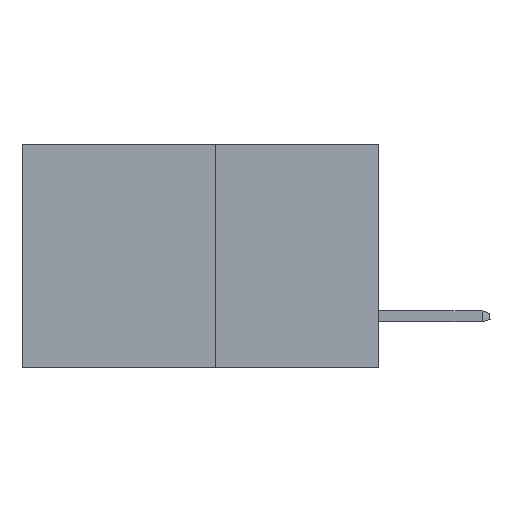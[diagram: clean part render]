
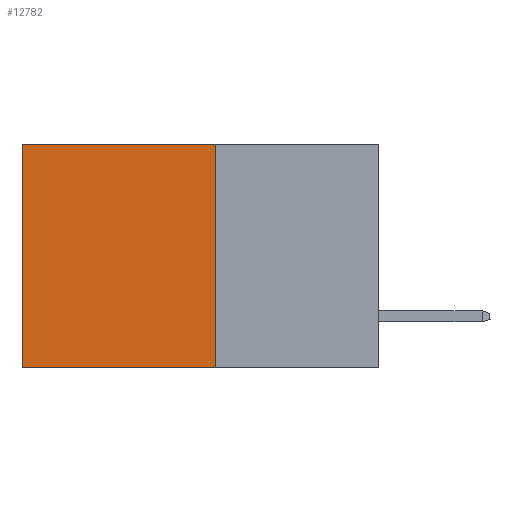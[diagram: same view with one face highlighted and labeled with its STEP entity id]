
A CAD part, left-side view. The second image highlights one B-rep face of the part: STEP entity #12782.
In plain terms, the highlighted planar face has unit normal (-1, 0, 0).
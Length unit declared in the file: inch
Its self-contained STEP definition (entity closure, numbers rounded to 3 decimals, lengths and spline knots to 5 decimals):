
#354 = VECTOR ( 'NONE', #17186, 39.37008 ) ;
#421 = EDGE_LOOP ( 'NONE', ( #5768, #6352, #7185, #8980 ) ) ;
#949 = VERTEX_POINT ( 'NONE', #8598 ) ;
#1017 = VERTEX_POINT ( 'NONE', #4522 ) ;
#3028 = LINE ( 'NONE', #9711, #18203 ) ;
#3648 = DIRECTION ( 'NONE',  ( 0., 0., -1. ) ) ;
#4522 = CARTESIAN_POINT ( 'NONE',  ( 0.277, 0.59, 0. ) ) ;
#4536 = VERTEX_POINT ( 'NONE', #15604 ) ;
#4765 = LINE ( 'NONE', #12818, #354 ) ;
#4774 = VECTOR ( 'NONE', #14787, 39.37008 ) ;
#5768 = ORIENTED_EDGE ( 'NONE', *, *, #16860, .T. ) ;
#6014 = CARTESIAN_POINT ( 'NONE',  ( 0.277, 0.27, 0. ) ) ;
#6352 = ORIENTED_EDGE ( 'NONE', *, *, #13840, .F. ) ;
#6993 = CARTESIAN_POINT ( 'NONE',  ( 0.277, 0.27, -0.37 ) ) ;
#7185 = ORIENTED_EDGE ( 'NONE', *, *, #7411, .F. ) ;
#7411 = EDGE_CURVE ( 'NONE', #949, #16861, #18290, .T. ) ;
#8253 = LINE ( 'NONE', #6014, #4774 ) ;
#8598 = CARTESIAN_POINT ( 'NONE',  ( 0.277, 0.27, 0. ) ) ;
#8980 = ORIENTED_EDGE ( 'NONE', *, *, #12491, .T. ) ;
#9711 = CARTESIAN_POINT ( 'NONE',  ( 0.277, 0.27, -0.37 ) ) ;
#10402 = DIRECTION ( 'NONE',  ( 0., 0., -1. ) ) ;
#10406 = CARTESIAN_POINT ( 'NONE',  ( 0.277, 0.27, -0.37 ) ) ;
#10921 = FACE_OUTER_BOUND ( 'NONE', #421, .T. ) ;
#10988 = VECTOR ( 'NONE', #10402, 39.37008 ) ;
#11010 = CARTESIAN_POINT ( 'NONE',  ( 0.277, 0.27, -0.37 ) ) ;
#12491 = EDGE_CURVE ( 'NONE', #949, #1017, #8253, .T. ) ;
#12495 = DIRECTION ( 'NONE',  ( 1., 0., 0. ) ) ;
#12782 = ADVANCED_FACE ( 'NONE', ( #10921 ), #16759, .F. ) ;
#12818 = CARTESIAN_POINT ( 'NONE',  ( 0.277, 0.59, -0.37 ) ) ;
#13840 = EDGE_CURVE ( 'NONE', #16861, #4536, #3028, .T. ) ;
#14097 = DIRECTION ( 'NONE',  ( 0., 1., 0. ) ) ;
#14787 = DIRECTION ( 'NONE',  ( 0., 1., 0. ) ) ;
#14793 = AXIS2_PLACEMENT_3D ( 'NONE', #11010, #12495, #3648 ) ;
#15604 = CARTESIAN_POINT ( 'NONE',  ( 0.277, 0.59, -0.37 ) ) ;
#16759 = PLANE ( 'NONE',  #14793 ) ;
#16860 = EDGE_CURVE ( 'NONE', #1017, #4536, #4765, .T. ) ;
#16861 = VERTEX_POINT ( 'NONE', #6993 ) ;
#17186 = DIRECTION ( 'NONE',  ( 0., 0., -1. ) ) ;
#18203 = VECTOR ( 'NONE', #14097, 39.37008 ) ;
#18290 = LINE ( 'NONE', #10406, #10988 ) ;
